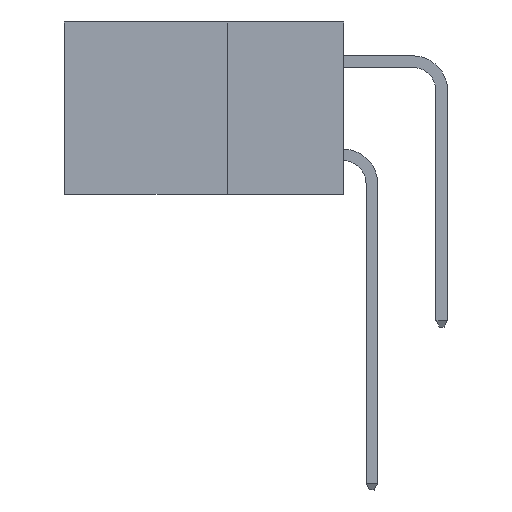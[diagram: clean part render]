
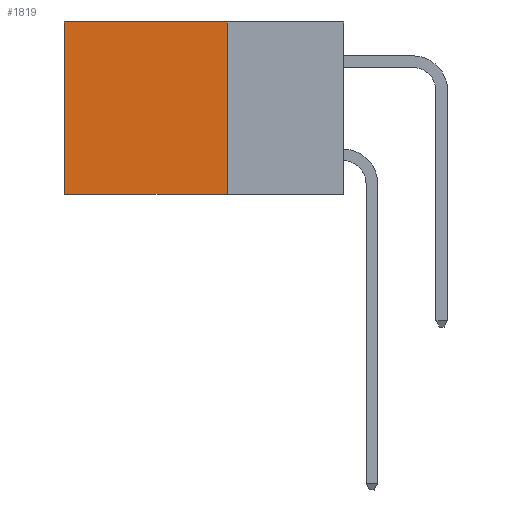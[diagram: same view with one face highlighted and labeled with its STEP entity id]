
A CAD part, left-side view. The second image highlights one B-rep face of the part: STEP entity #1819.
In plain terms, the highlighted planar face has unit normal (-1, 0, 0).
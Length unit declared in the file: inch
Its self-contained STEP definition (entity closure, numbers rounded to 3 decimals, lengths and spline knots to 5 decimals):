
#696 = EDGE_CURVE ( 'NONE', #17771, #10381, #19894, .T. ) ;
#1030 = VECTOR ( 'NONE', #15229, 39.37008 ) ;
#1160 = LINE ( 'NONE', #23849, #20913 ) ;
#1551 = CARTESIAN_POINT ( 'NONE',  ( 0.2615, 0.6, 0. ) ) ;
#1819 = ADVANCED_FACE ( 'NONE', ( #21957 ), #8685, .F. ) ;
#1889 = EDGE_CURVE ( 'NONE', #4685, #10381, #1160, .T. ) ;
#4005 = EDGE_LOOP ( 'NONE', ( #12208, #12148, #14963, #19581 ) ) ;
#4685 = VERTEX_POINT ( 'NONE', #13357 ) ;
#6551 = CARTESIAN_POINT ( 'NONE',  ( 0.2615, 0.25, -0.37 ) ) ;
#8515 = VECTOR ( 'NONE', #11518, 39.37008 ) ;
#8685 = PLANE ( 'NONE',  #24123 ) ;
#9598 = CARTESIAN_POINT ( 'NONE',  ( 0.2615, 0.25, 0. ) ) ;
#10132 = EDGE_CURVE ( 'NONE', #15561, #4685, #20686, .T. ) ;
#10381 = VERTEX_POINT ( 'NONE', #10760 ) ;
#10694 = DIRECTION ( 'NONE',  ( 0., 1., 0. ) ) ;
#10760 = CARTESIAN_POINT ( 'NONE',  ( 0.2615, 0.6, -0.37 ) ) ;
#11235 = LINE ( 'NONE', #9598, #1030 ) ;
#11518 = DIRECTION ( 'NONE',  ( 0., 0., -1. ) ) ;
#12148 = ORIENTED_EDGE ( 'NONE', *, *, #1889, .F. ) ;
#12208 = ORIENTED_EDGE ( 'NONE', *, *, #696, .T. ) ;
#13357 = CARTESIAN_POINT ( 'NONE',  ( 0.2615, 0.25, -0.37 ) ) ;
#13764 = DIRECTION ( 'NONE',  ( 0., 0., -1. ) ) ;
#13768 = EDGE_CURVE ( 'NONE', #15561, #17771, #11235, .T. ) ;
#14688 = DIRECTION ( 'NONE',  ( 1., 0., 0. ) ) ;
#14963 = ORIENTED_EDGE ( 'NONE', *, *, #10132, .F. ) ;
#15229 = DIRECTION ( 'NONE',  ( 0., 1., 0. ) ) ;
#15561 = VERTEX_POINT ( 'NONE', #20520 ) ;
#16417 = DIRECTION ( 'NONE',  ( 0., 0., -1. ) ) ;
#16898 = CARTESIAN_POINT ( 'NONE',  ( 0.2615, 0.25, -0.37 ) ) ;
#17771 = VERTEX_POINT ( 'NONE', #1551 ) ;
#19581 = ORIENTED_EDGE ( 'NONE', *, *, #13768, .T. ) ;
#19894 = LINE ( 'NONE', #21529, #23451 ) ;
#20520 = CARTESIAN_POINT ( 'NONE',  ( 0.2615, 0.25, 0. ) ) ;
#20686 = LINE ( 'NONE', #16898, #8515 ) ;
#20913 = VECTOR ( 'NONE', #10694, 39.37008 ) ;
#21529 = CARTESIAN_POINT ( 'NONE',  ( 0.2615, 0.6, -0.37 ) ) ;
#21957 = FACE_OUTER_BOUND ( 'NONE', #4005, .T. ) ;
#23451 = VECTOR ( 'NONE', #13764, 39.37008 ) ;
#23849 = CARTESIAN_POINT ( 'NONE',  ( 0.2615, 0.25, -0.37 ) ) ;
#24123 = AXIS2_PLACEMENT_3D ( 'NONE', #6551, #14688, #16417 ) ;
